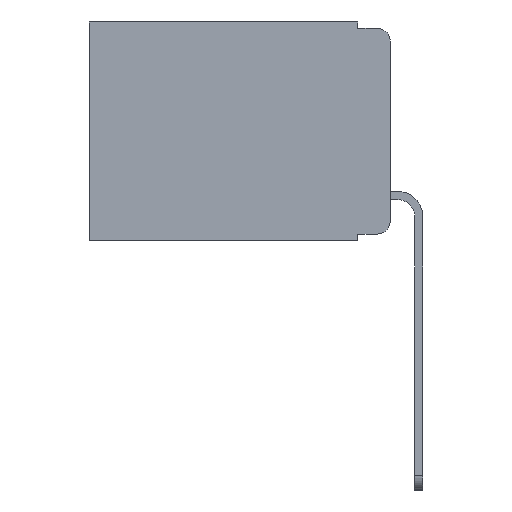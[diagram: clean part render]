
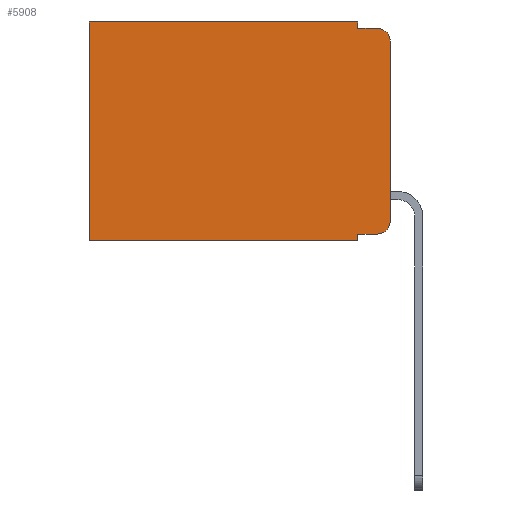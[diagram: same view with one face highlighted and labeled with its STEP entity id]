
A CAD part, left-side view. The second image highlights one B-rep face of the part: STEP entity #5908.
In plain terms, the highlighted planar face has unit normal (-1, 0, 0).
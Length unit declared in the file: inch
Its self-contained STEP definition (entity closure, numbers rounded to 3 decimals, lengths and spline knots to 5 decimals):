
#231 = CARTESIAN_POINT ( 'NONE',  ( 0.298, 0.02, -0.01 ) ) ;
#288 = EDGE_LOOP ( 'NONE', ( #10118, #7321, #6963, #2082, #2497, #9333, #2931, #10527, #2053, #1498 ) ) ;
#311 = CARTESIAN_POINT ( 'NONE',  ( 0.298, 0.051, -0.01 ) ) ;
#555 = VECTOR ( 'NONE', #3875, 39.37008 ) ;
#953 = CIRCLE ( 'NONE', #2650, 0.02 ) ;
#1081 = EDGE_CURVE ( 'NONE', #4850, #6052, #6314, .T. ) ;
#1089 = VECTOR ( 'NONE', #5464, 39.37008 ) ;
#1437 = LINE ( 'NONE', #6511, #1089 ) ;
#1498 = ORIENTED_EDGE ( 'NONE', *, *, #11543, .T. ) ;
#1794 = CARTESIAN_POINT ( 'NONE',  ( 0.298, 0.051, 0. ) ) ;
#2053 = ORIENTED_EDGE ( 'NONE', *, *, #7397, .T. ) ;
#2082 = ORIENTED_EDGE ( 'NONE', *, *, #11633, .F. ) ;
#2217 = LINE ( 'NONE', #11301, #4313 ) ;
#2497 = ORIENTED_EDGE ( 'NONE', *, *, #12252, .T. ) ;
#2533 = EDGE_CURVE ( 'NONE', #12261, #7528, #3432, .T. ) ;
#2650 = AXIS2_PLACEMENT_3D ( 'NONE', #9302, #5207, #6128 ) ;
#2808 = DIRECTION ( 'NONE',  ( 0., 0., -1. ) ) ;
#2931 = ORIENTED_EDGE ( 'NONE', *, *, #2533, .F. ) ;
#3190 = CARTESIAN_POINT ( 'NONE',  ( 0.298, 0., 0. ) ) ;
#3432 = LINE ( 'NONE', #9403, #10898 ) ;
#3741 = CARTESIAN_POINT ( 'NONE',  ( 0.298, 0., 0. ) ) ;
#3875 = DIRECTION ( 'NONE',  ( 0., 1., 0. ) ) ;
#4119 = VERTEX_POINT ( 'NONE', #10052 ) ;
#4193 = DIRECTION ( 'NONE',  ( 0., 0., -1. ) ) ;
#4313 = VECTOR ( 'NONE', #7306, 39.37008 ) ;
#4667 = CARTESIAN_POINT ( 'NONE',  ( 0.298, 0.02, -0.333 ) ) ;
#4676 = LINE ( 'NONE', #5672, #555 ) ;
#4850 = VERTEX_POINT ( 'NONE', #10809 ) ;
#5207 = DIRECTION ( 'NONE',  ( -1., 0., 0. ) ) ;
#5456 = LINE ( 'NONE', #11677, #8711 ) ;
#5464 = DIRECTION ( 'NONE',  ( 0., 0., -1. ) ) ;
#5672 = CARTESIAN_POINT ( 'NONE',  ( 0.298, 0., 0. ) ) ;
#5682 = EDGE_CURVE ( 'NONE', #4119, #12261, #1437, .T. ) ;
#5908 = ADVANCED_FACE ( 'NONE', ( #8766 ), #10909, .F. ) ;
#6040 = CARTESIAN_POINT ( 'NONE',  ( 0.298, 0.473, 0. ) ) ;
#6052 = VERTEX_POINT ( 'NONE', #231 ) ;
#6128 = DIRECTION ( 'NONE',  ( 0., 0., -1. ) ) ;
#6314 = CIRCLE ( 'NONE', #6730, 0.02 ) ;
#6511 = CARTESIAN_POINT ( 'NONE',  ( 0.298, 0.051, 0. ) ) ;
#6730 = AXIS2_PLACEMENT_3D ( 'NONE', #12498, #9578, #8575 ) ;
#6963 = ORIENTED_EDGE ( 'NONE', *, *, #10214, .F. ) ;
#6965 = DIRECTION ( 'NONE',  ( 1., 0., 0. ) ) ;
#7029 = VERTEX_POINT ( 'NONE', #4667 ) ;
#7088 = DIRECTION ( 'NONE',  ( 0., 0., -1. ) ) ;
#7306 = DIRECTION ( 'NONE',  ( 0., -1., 0. ) ) ;
#7321 = ORIENTED_EDGE ( 'NONE', *, *, #1081, .T. ) ;
#7397 = EDGE_CURVE ( 'NONE', #4119, #7029, #5456, .T. ) ;
#7528 = VERTEX_POINT ( 'NONE', #11023 ) ;
#7768 = CARTESIAN_POINT ( 'NONE',  ( 0.298, 0.051, -0.343 ) ) ;
#8113 = VECTOR ( 'NONE', #4193, 39.37008 ) ;
#8575 = DIRECTION ( 'NONE',  ( 0., 0., -1. ) ) ;
#8711 = VECTOR ( 'NONE', #11481, 39.37008 ) ;
#8766 = FACE_OUTER_BOUND ( 'NONE', #288, .T. ) ;
#9302 = CARTESIAN_POINT ( 'NONE',  ( 0.298, 0.02, -0.313 ) ) ;
#9333 = ORIENTED_EDGE ( 'NONE', *, *, #10655, .T. ) ;
#9403 = CARTESIAN_POINT ( 'NONE',  ( 0.298, 0., -0.343 ) ) ;
#9535 = DIRECTION ( 'NONE',  ( 0., 1., 0. ) ) ;
#9578 = DIRECTION ( 'NONE',  ( -1., 0., 0. ) ) ;
#9966 = AXIS2_PLACEMENT_3D ( 'NONE', #3741, #6965, #2808 ) ;
#10052 = CARTESIAN_POINT ( 'NONE',  ( 0.298, 0.051, -0.333 ) ) ;
#10118 = ORIENTED_EDGE ( 'NONE', *, *, #10674, .F. ) ;
#10214 = EDGE_CURVE ( 'NONE', #12654, #6052, #2217, .T. ) ;
#10297 = LINE ( 'NONE', #6040, #12996 ) ;
#10485 = VECTOR ( 'NONE', #11871, 39.37008 ) ;
#10527 = ORIENTED_EDGE ( 'NONE', *, *, #5682, .F. ) ;
#10580 = CARTESIAN_POINT ( 'NONE',  ( 0.298, 0.473, 0. ) ) ;
#10655 = EDGE_CURVE ( 'NONE', #12142, #7528, #10297, .T. ) ;
#10674 = EDGE_CURVE ( 'NONE', #4850, #12858, #12217, .T. ) ;
#10809 = CARTESIAN_POINT ( 'NONE',  ( 0.298, 0., -0.03 ) ) ;
#10898 = VECTOR ( 'NONE', #9535, 39.37008 ) ;
#10909 = PLANE ( 'NONE',  #9966 ) ;
#11023 = CARTESIAN_POINT ( 'NONE',  ( 0.298, 0.473, -0.343 ) ) ;
#11301 = CARTESIAN_POINT ( 'NONE',  ( 0.298, 0.051, -0.01 ) ) ;
#11481 = DIRECTION ( 'NONE',  ( 0., -1., 0. ) ) ;
#11543 = EDGE_CURVE ( 'NONE', #7029, #12858, #953, .T. ) ;
#11633 = EDGE_CURVE ( 'NONE', #13017, #12654, #12870, .T. ) ;
#11677 = CARTESIAN_POINT ( 'NONE',  ( 0.298, 0.051, -0.333 ) ) ;
#11871 = DIRECTION ( 'NONE',  ( 0., 0., -1. ) ) ;
#12142 = VERTEX_POINT ( 'NONE', #10580 ) ;
#12217 = LINE ( 'NONE', #3190, #8113 ) ;
#12219 = CARTESIAN_POINT ( 'NONE',  ( 0.298, 0., -0.313 ) ) ;
#12252 = EDGE_CURVE ( 'NONE', #13017, #12142, #4676, .T. ) ;
#12261 = VERTEX_POINT ( 'NONE', #7768 ) ;
#12498 = CARTESIAN_POINT ( 'NONE',  ( 0.298, 0.02, -0.03 ) ) ;
#12602 = CARTESIAN_POINT ( 'NONE',  ( 0.298, 0.051, 0. ) ) ;
#12654 = VERTEX_POINT ( 'NONE', #311 ) ;
#12858 = VERTEX_POINT ( 'NONE', #12219 ) ;
#12870 = LINE ( 'NONE', #1794, #10485 ) ;
#12996 = VECTOR ( 'NONE', #7088, 39.37008 ) ;
#13017 = VERTEX_POINT ( 'NONE', #12602 ) ;
